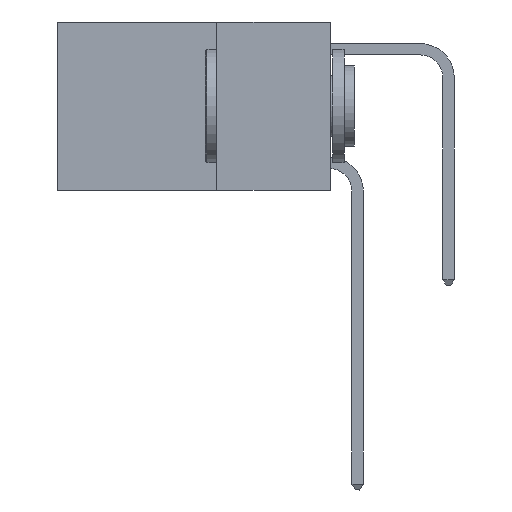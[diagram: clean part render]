
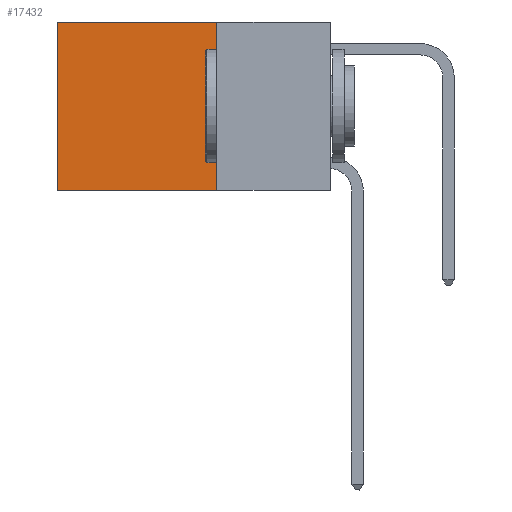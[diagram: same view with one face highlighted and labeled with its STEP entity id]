
A CAD part, left-side view. The second image highlights one B-rep face of the part: STEP entity #17432.
In plain terms, the highlighted planar face has unit normal (-1, 0, 0).
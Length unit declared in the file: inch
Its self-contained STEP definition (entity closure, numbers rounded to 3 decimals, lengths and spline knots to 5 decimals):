
#541 = DIRECTION ( 'NONE',  ( 0., 0., -1. ) ) ;
#860 = LINE ( 'NONE', #30215, #3235 ) ;
#1682 = DIRECTION ( 'NONE',  ( 0., 1., 0. ) ) ;
#3235 = VECTOR ( 'NONE', #541, 39.37008 ) ;
#3702 = VERTEX_POINT ( 'NONE', #7543 ) ;
#4401 = LINE ( 'NONE', #31494, #9280 ) ;
#4609 = EDGE_LOOP ( 'NONE', ( #12687, #13445, #24495, #26218 ) ) ;
#4969 = FACE_OUTER_BOUND ( 'NONE', #4609, .T. ) ;
#5049 = VERTEX_POINT ( 'NONE', #5611 ) ;
#5611 = CARTESIAN_POINT ( 'NONE',  ( 0.2625, 0.25, -0.37 ) ) ;
#6516 = DIRECTION ( 'NONE',  ( 0., 0., -1. ) ) ;
#6658 = VERTEX_POINT ( 'NONE', #23320 ) ;
#7543 = CARTESIAN_POINT ( 'NONE',  ( 0.2625, 0.6, -0.37 ) ) ;
#9280 = VECTOR ( 'NONE', #6516, 39.37008 ) ;
#10049 = EDGE_CURVE ( 'NONE', #6658, #3702, #860, .T. ) ;
#12006 = CARTESIAN_POINT ( 'NONE',  ( 0.2625, 0.25, 0. ) ) ;
#12687 = ORIENTED_EDGE ( 'NONE', *, *, #10049, .T. ) ;
#13445 = ORIENTED_EDGE ( 'NONE', *, *, #14212, .F. ) ;
#14212 = EDGE_CURVE ( 'NONE', #5049, #3702, #21333, .T. ) ;
#14961 = VECTOR ( 'NONE', #31230, 39.37008 ) ;
#17432 = ADVANCED_FACE ( 'NONE', ( #4969 ), #24942, .F. ) ;
#18761 = CARTESIAN_POINT ( 'NONE',  ( 0.2625, 0.25, -0.37 ) ) ;
#19950 = CARTESIAN_POINT ( 'NONE',  ( 0.2625, 0.25, 0. ) ) ;
#19955 = AXIS2_PLACEMENT_3D ( 'NONE', #19950, #22542, #29805 ) ;
#20998 = VERTEX_POINT ( 'NONE', #22593 ) ;
#21333 = LINE ( 'NONE', #18761, #28651 ) ;
#22542 = DIRECTION ( 'NONE',  ( 1., 0., 0. ) ) ;
#22593 = CARTESIAN_POINT ( 'NONE',  ( 0.2625, 0.25, 0. ) ) ;
#23320 = CARTESIAN_POINT ( 'NONE',  ( 0.2625, 0.6, 0. ) ) ;
#24495 = ORIENTED_EDGE ( 'NONE', *, *, #25782, .F. ) ;
#24942 = PLANE ( 'NONE',  #19955 ) ;
#25782 = EDGE_CURVE ( 'NONE', #20998, #5049, #4401, .T. ) ;
#26218 = ORIENTED_EDGE ( 'NONE', *, *, #26820, .T. ) ;
#26820 = EDGE_CURVE ( 'NONE', #20998, #6658, #28961, .T. ) ;
#28651 = VECTOR ( 'NONE', #1682, 39.37008 ) ;
#28961 = LINE ( 'NONE', #12006, #14961 ) ;
#29805 = DIRECTION ( 'NONE',  ( 0., 0., -1. ) ) ;
#30215 = CARTESIAN_POINT ( 'NONE',  ( 0.2625, 0.6, 0. ) ) ;
#31230 = DIRECTION ( 'NONE',  ( 0., 1., 0. ) ) ;
#31494 = CARTESIAN_POINT ( 'NONE',  ( 0.2625, 0.25, 0. ) ) ;
